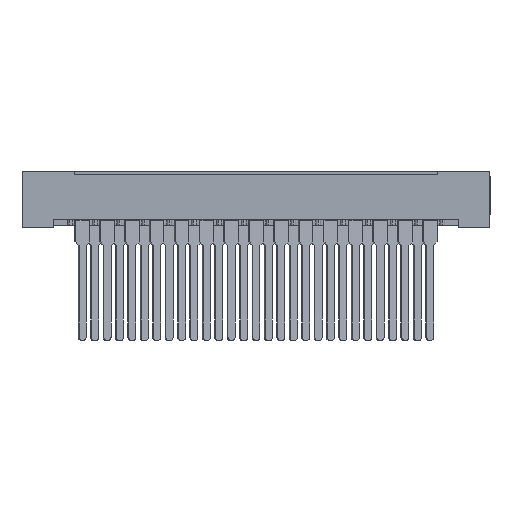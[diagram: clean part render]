
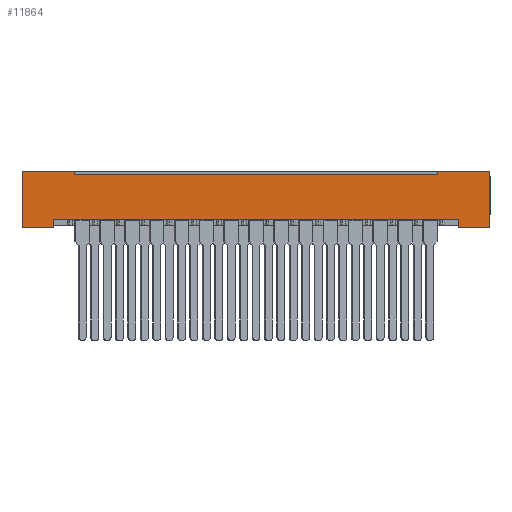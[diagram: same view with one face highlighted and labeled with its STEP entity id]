
A CAD part, top view. The second image highlights one B-rep face of the part: STEP entity #11864.
In plain terms, the highlighted planar face has unit normal (0, 0, 1).
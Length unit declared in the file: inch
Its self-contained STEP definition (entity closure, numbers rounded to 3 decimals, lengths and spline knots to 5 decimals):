
#181 = ORIENTED_EDGE ( 'NONE', *, *, #14503, .T. ) ;
#509 = VERTEX_POINT ( 'NONE', #6169 ) ;
#673 = VECTOR ( 'NONE', #10990, 39.37008 ) ;
#733 = DIRECTION ( 'NONE',  ( 1., 0., 0. ) ) ;
#749 = VERTEX_POINT ( 'NONE', #11431 ) ;
#875 = DIRECTION ( 'NONE',  ( 0., -1., 0. ) ) ;
#959 = VERTEX_POINT ( 'NONE', #5943 ) ;
#1105 = VERTEX_POINT ( 'NONE', #4870 ) ;
#1199 = LINE ( 'NONE', #10523, #1450 ) ;
#1450 = VECTOR ( 'NONE', #15156, 39.37008 ) ;
#1614 = VECTOR ( 'NONE', #875, 39.37008 ) ;
#1632 = ORIENTED_EDGE ( 'NONE', *, *, #13616, .T. ) ;
#1848 = LINE ( 'NONE', #20075, #1614 ) ;
#2313 = CARTESIAN_POINT ( 'NONE',  ( 0., 0.453, 0. ) ) ;
#2630 = VECTOR ( 'NONE', #5981, 39.37008 ) ;
#2975 = ORIENTED_EDGE ( 'NONE', *, *, #11161, .F. ) ;
#2989 = ORIENTED_EDGE ( 'NONE', *, *, #16919, .T. ) ;
#3266 = EDGE_CURVE ( 'NONE', #18245, #18286, #18869, .T. ) ;
#4247 = ORIENTED_EDGE ( 'NONE', *, *, #20067, .F. ) ;
#4544 = CARTESIAN_POINT ( 'NONE',  ( 3.77, 0.453, 0. ) ) ;
#4573 = CARTESIAN_POINT ( 'NONE',  ( 0.42, 0.423, 0. ) ) ;
#4596 = EDGE_CURVE ( 'NONE', #9501, #509, #1848, .T. ) ;
#4737 = LINE ( 'NONE', #11460, #10305 ) ;
#4870 = CARTESIAN_POINT ( 'NONE',  ( 3.52, 0.062, 0. ) ) ;
#4939 = VERTEX_POINT ( 'NONE', #19439 ) ;
#5156 = CARTESIAN_POINT ( 'NONE',  ( 0., 0.423, 0. ) ) ;
#5261 = EDGE_CURVE ( 'NONE', #4939, #509, #12509, .T. ) ;
#5368 = CARTESIAN_POINT ( 'NONE',  ( 0., 0., 0. ) ) ;
#5943 = CARTESIAN_POINT ( 'NONE',  ( 0.42, 0.453, 0. ) ) ;
#5981 = DIRECTION ( 'NONE',  ( 1., 0., 0. ) ) ;
#6169 = CARTESIAN_POINT ( 'NONE',  ( 0.25, 0., 0. ) ) ;
#6234 = LINE ( 'NONE', #9448, #11588 ) ;
#6383 = VERTEX_POINT ( 'NONE', #6524 ) ;
#6524 = CARTESIAN_POINT ( 'NONE',  ( 3.77, 0., 0. ) ) ;
#6947 = CARTESIAN_POINT ( 'NONE',  ( 0.25, 0.062, 0. ) ) ;
#6959 = ORIENTED_EDGE ( 'NONE', *, *, #4596, .F. ) ;
#7166 = EDGE_CURVE ( 'NONE', #14843, #959, #17079, .T. ) ;
#7373 = VERTEX_POINT ( 'NONE', #7899 ) ;
#7604 = LINE ( 'NONE', #19329, #11925 ) ;
#7631 = CARTESIAN_POINT ( 'NONE',  ( 0.42, 0.423, 0. ) ) ;
#7718 = VECTOR ( 'NONE', #18197, 39.37008 ) ;
#7899 = CARTESIAN_POINT ( 'NONE',  ( 3.52, 0., 0. ) ) ;
#8672 = EDGE_LOOP ( 'NONE', ( #4247, #181, #1632, #14802, #2975, #17762, #17791, #16790, #10070, #2989, #12066, #6959 ) ) ;
#9168 = EDGE_CURVE ( 'NONE', #18245, #959, #14215, .T. ) ;
#9219 = VECTOR ( 'NONE', #15914, 39.37008 ) ;
#9223 = FACE_OUTER_BOUND ( 'NONE', #8672, .T. ) ;
#9424 = VECTOR ( 'NONE', #9549, 39.37008 ) ;
#9448 = CARTESIAN_POINT ( 'NONE',  ( 0., 0.453, 0. ) ) ;
#9469 = CARTESIAN_POINT ( 'NONE',  ( 0., 0.453, 0. ) ) ;
#9501 = VERTEX_POINT ( 'NONE', #6947 ) ;
#9549 = DIRECTION ( 'NONE',  ( 1., 0., 0. ) ) ;
#9670 = DIRECTION ( 'NONE',  ( 0., -1., 0. ) ) ;
#9973 = EDGE_CURVE ( 'NONE', #18286, #749, #4737, .T. ) ;
#10070 = ORIENTED_EDGE ( 'NONE', *, *, #7166, .F. ) ;
#10251 = PLANE ( 'NONE',  #13271 ) ;
#10305 = VECTOR ( 'NONE', #13308, 39.37008 ) ;
#10382 = DIRECTION ( 'NONE',  ( -1., 0., 0. ) ) ;
#10452 = DIRECTION ( 'NONE',  ( 0., 0., -1. ) ) ;
#10523 = CARTESIAN_POINT ( 'NONE',  ( 0., 0.062, 0. ) ) ;
#10639 = LINE ( 'NONE', #11470, #19745 ) ;
#10678 = CARTESIAN_POINT ( 'NONE',  ( 3.35, 0.423, 0. ) ) ;
#10990 = DIRECTION ( 'NONE',  ( 0., -1., 0. ) ) ;
#11161 = EDGE_CURVE ( 'NONE', #749, #15212, #6234, .T. ) ;
#11431 = CARTESIAN_POINT ( 'NONE',  ( 3.35, 0.453, 0. ) ) ;
#11460 = CARTESIAN_POINT ( 'NONE',  ( 3.35, 0.423, 0. ) ) ;
#11470 = CARTESIAN_POINT ( 'NONE',  ( 3.52, 0.017, 0. ) ) ;
#11588 = VECTOR ( 'NONE', #16325, 39.37008 ) ;
#11707 = LINE ( 'NONE', #5368, #15003 ) ;
#11864 = ADVANCED_FACE ( 'NONE', ( #9223 ), #10251, .F. ) ;
#11925 = VECTOR ( 'NONE', #16113, 39.37008 ) ;
#12066 = ORIENTED_EDGE ( 'NONE', *, *, #5261, .T. ) ;
#12509 = LINE ( 'NONE', #15768, #2630 ) ;
#13271 = AXIS2_PLACEMENT_3D ( 'NONE', #20068, #10452, #10382 ) ;
#13308 = DIRECTION ( 'NONE',  ( 0., 1., 0. ) ) ;
#13616 = EDGE_CURVE ( 'NONE', #7373, #6383, #11707, .T. ) ;
#14215 = LINE ( 'NONE', #4573, #9219 ) ;
#14503 = EDGE_CURVE ( 'NONE', #1105, #7373, #10639, .T. ) ;
#14802 = ORIENTED_EDGE ( 'NONE', *, *, #19681, .F. ) ;
#14843 = VERTEX_POINT ( 'NONE', #2313 ) ;
#15003 = VECTOR ( 'NONE', #733, 39.37008 ) ;
#15156 = DIRECTION ( 'NONE',  ( -1., 0., 0. ) ) ;
#15212 = VERTEX_POINT ( 'NONE', #17941 ) ;
#15768 = CARTESIAN_POINT ( 'NONE',  ( 0., 0., 0. ) ) ;
#15914 = DIRECTION ( 'NONE',  ( 0., 1., 0. ) ) ;
#16113 = DIRECTION ( 'NONE',  ( 0., -1., 0. ) ) ;
#16124 = LINE ( 'NONE', #4544, #673 ) ;
#16325 = DIRECTION ( 'NONE',  ( 1., 0., 0. ) ) ;
#16790 = ORIENTED_EDGE ( 'NONE', *, *, #9168, .T. ) ;
#16919 = EDGE_CURVE ( 'NONE', #14843, #4939, #7604, .T. ) ;
#17079 = LINE ( 'NONE', #9469, #9424 ) ;
#17762 = ORIENTED_EDGE ( 'NONE', *, *, #9973, .F. ) ;
#17791 = ORIENTED_EDGE ( 'NONE', *, *, #3266, .F. ) ;
#17941 = CARTESIAN_POINT ( 'NONE',  ( 3.77, 0.453, 0. ) ) ;
#18197 = DIRECTION ( 'NONE',  ( 1., 0., 0. ) ) ;
#18245 = VERTEX_POINT ( 'NONE', #7631 ) ;
#18286 = VERTEX_POINT ( 'NONE', #10678 ) ;
#18869 = LINE ( 'NONE', #5156, #7718 ) ;
#19329 = CARTESIAN_POINT ( 'NONE',  ( 0., 0.453, 0. ) ) ;
#19439 = CARTESIAN_POINT ( 'NONE',  ( 0., 0., 0. ) ) ;
#19681 = EDGE_CURVE ( 'NONE', #15212, #6383, #16124, .T. ) ;
#19745 = VECTOR ( 'NONE', #9670, 39.37008 ) ;
#20067 = EDGE_CURVE ( 'NONE', #1105, #9501, #1199, .T. ) ;
#20068 = CARTESIAN_POINT ( 'NONE',  ( 0., 0.453, 0. ) ) ;
#20075 = CARTESIAN_POINT ( 'NONE',  ( 0.25, 0.017, 0. ) ) ;
